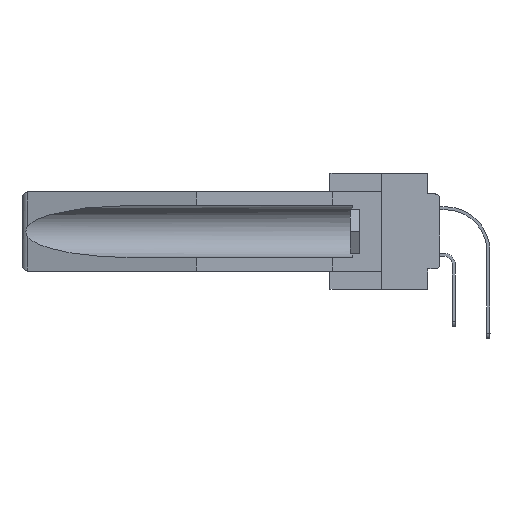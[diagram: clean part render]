
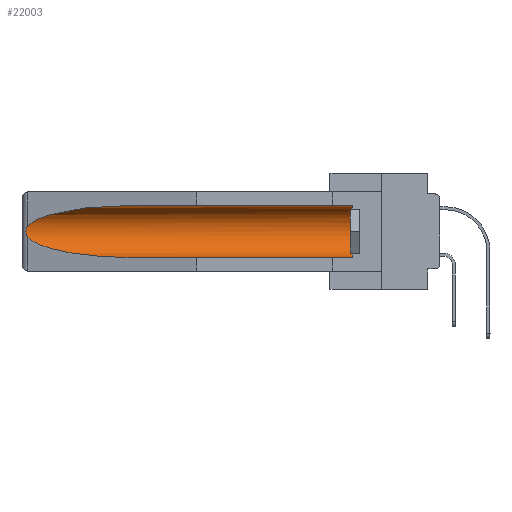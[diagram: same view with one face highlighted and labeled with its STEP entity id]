
A CAD part, left-side view. The second image highlights one B-rep face of the part: STEP entity #22003.
In plain terms, the highlighted cylindrical face has radius 2.857 mm (diameter 5.715 mm), a partial arc.
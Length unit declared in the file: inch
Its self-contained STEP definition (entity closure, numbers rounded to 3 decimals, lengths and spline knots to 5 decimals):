
#456 = AXIS2_PLACEMENT_3D ( 'NONE', #16106, #8816, #16276 ) ;
#2044 =( BOUNDED_CURVE ( )  B_SPLINE_CURVE ( 3, ( #31235, #7769, #9814, #15415 ),
 .UNSPECIFIED., .F., .T. ) 
 B_SPLINE_CURVE_WITH_KNOTS ( ( 4, 4 ),
 ( 0.1948, 1.5708 ),
 .UNSPECIFIED. ) 
 CURVE ( )  GEOMETRIC_REPRESENTATION_ITEM ( )  RATIONAL_B_SPLINE_CURVE ( ( 1., 0.848, 0.848, 1. ) ) 
 REPRESENTATION_ITEM ( '' )  );
#2384 = CARTESIAN_POINT ( 'NONE',  ( 0.26597, 1.52961, -0.15275 ) ) ;
#2824 = CARTESIAN_POINT ( 'NONE',  ( 0.155, 0.126, -0.284 ) ) ;
#3702 = EDGE_CURVE ( 'NONE', #22086, #7936, #31306, .T. ) ;
#4002 = CARTESIAN_POINT ( 'NONE',  ( 0.25451, 1.48313, -0.09465 ) ) ;
#5752 = DIRECTION ( 'NONE',  ( 0., 1., 0. ) ) ;
#6149 = ORIENTED_EDGE ( 'NONE', *, *, #23588, .T. ) ;
#6711 = ORIENTED_EDGE ( 'NONE', *, *, #3702, .F. ) ;
#6975 = CIRCLE ( 'NONE', #456, 0.1125 ) ;
#7311 = CARTESIAN_POINT ( 'NONE',  ( 0.26537, 1.52718, -0.19328 ) ) ;
#7769 = CARTESIAN_POINT ( 'NONE',  ( 0.25451, 1.48313, -0.24835 ) ) ;
#7911 =( BOUNDED_CURVE ( )  B_SPLINE_CURVE ( 3, ( #32397, #29522, #4002, #13861 ),
 .UNSPECIFIED., .F., .T. ) 
 B_SPLINE_CURVE_WITH_KNOTS ( ( 4, 4 ),
 ( 4.71239, 6.08839 ),
 .UNSPECIFIED. ) 
 CURVE ( )  GEOMETRIC_REPRESENTATION_ITEM ( )  RATIONAL_B_SPLINE_CURVE ( ( 1., 0.848, 0.848, 1. ) ) 
 REPRESENTATION_ITEM ( '' )  );
#7936 = VERTEX_POINT ( 'NONE', #20346 ) ;
#8816 = DIRECTION ( 'NONE',  ( 0., -1., 0. ) ) ;
#9614 = B_SPLINE_CURVE_WITH_KNOTS ( 'NONE', 3,
 ( #25510, #2384, #25689, #17685, #12581, #9988, #33340, #15611, #12745, #31127 ),
 .UNSPECIFIED., .F., .F.,
 ( 4, 2, 2, 2, 4 ),
 ( 0., 0.00029, 0.00058, 0.00087, 0.00117 ),
 .UNSPECIFIED. ) ;
#9814 = CARTESIAN_POINT ( 'NONE',  ( 0.21114, 1.30732, -0.284 ) ) ;
#9988 = CARTESIAN_POINT ( 'NONE',  ( 0.2675, 1.53308, -0.17534 ) ) ;
#11127 = VERTEX_POINT ( 'NONE', #25170 ) ;
#12581 = CARTESIAN_POINT ( 'NONE',  ( 0.2675, 1.53308, -0.16763 ) ) ;
#12745 = CARTESIAN_POINT ( 'NONE',  ( 0.26597, 1.5296, -0.19026 ) ) ;
#13861 = CARTESIAN_POINT ( 'NONE',  ( 0.26537, 1.52718, -0.14972 ) ) ;
#14024 = AXIS2_PLACEMENT_3D ( 'NONE', #25634, #17460, #25299 ) ;
#15058 = VECTOR ( 'NONE', #26028, 39.37008 ) ;
#15144 = EDGE_CURVE ( 'NONE', #23398, #25483, #9614, .T. ) ;
#15415 = CARTESIAN_POINT ( 'NONE',  ( 0.155, 1.07973, -0.284 ) ) ;
#15570 = CARTESIAN_POINT ( 'NONE',  ( 0.26537, 1.52718, -0.14972 ) ) ;
#15611 = CARTESIAN_POINT ( 'NONE',  ( 0.26655, 1.53094, -0.18657 ) ) ;
#15636 = CARTESIAN_POINT ( 'NONE',  ( 0.155, -0.30754, -0.284 ) ) ;
#16106 = CARTESIAN_POINT ( 'NONE',  ( 0.155, 0.126, -0.1715 ) ) ;
#16193 = VECTOR ( 'NONE', #5752, 39.37008 ) ;
#16276 = DIRECTION ( 'NONE',  ( 0., 0., 1. ) ) ;
#17460 = DIRECTION ( 'NONE',  ( 0., 1., 0. ) ) ;
#17685 = CARTESIAN_POINT ( 'NONE',  ( 0.2673, 1.5327, -0.16383 ) ) ;
#19900 = ORIENTED_EDGE ( 'NONE', *, *, #15144, .T. ) ;
#20346 = CARTESIAN_POINT ( 'NONE',  ( 0.155, 1.07973, -0.284 ) ) ;
#21026 = VERTEX_POINT ( 'NONE', #28425 ) ;
#21046 = LINE ( 'NONE', #23953, #16193 ) ;
#21612 = EDGE_CURVE ( 'NONE', #21026, #11127, #21046, .T. ) ;
#22003 = ADVANCED_FACE ( 'NONE', ( #27672 ), #24957, .F. ) ;
#22086 = VERTEX_POINT ( 'NONE', #2824 ) ;
#23398 = VERTEX_POINT ( 'NONE', #15570 ) ;
#23588 = EDGE_CURVE ( 'NONE', #11127, #23398, #7911, .T. ) ;
#23953 = CARTESIAN_POINT ( 'NONE',  ( 0.155, -0.30754, -0.059 ) ) ;
#24957 = CYLINDRICAL_SURFACE ( 'NONE', #14024, 0.1125 ) ;
#25170 = CARTESIAN_POINT ( 'NONE',  ( 0.155, 1.07973, -0.059 ) ) ;
#25299 = DIRECTION ( 'NONE',  ( 0., 0., 1. ) ) ;
#25483 = VERTEX_POINT ( 'NONE', #7311 ) ;
#25510 = CARTESIAN_POINT ( 'NONE',  ( 0.26537, 1.52718, -0.14972 ) ) ;
#25634 = CARTESIAN_POINT ( 'NONE',  ( 0.155, -0.30754, -0.1715 ) ) ;
#25689 = CARTESIAN_POINT ( 'NONE',  ( 0.26654, 1.53092, -0.15636 ) ) ;
#25864 = EDGE_CURVE ( 'NONE', #25483, #7936, #2044, .T. ) ;
#26015 = ORIENTED_EDGE ( 'NONE', *, *, #21612, .T. ) ;
#26028 = DIRECTION ( 'NONE',  ( 0., 1., 0. ) ) ;
#27672 = FACE_OUTER_BOUND ( 'NONE', #28005, .T. ) ;
#28005 = EDGE_LOOP ( 'NONE', ( #6149, #19900, #28353, #6711, #31223, #26015 ) ) ;
#28340 = EDGE_CURVE ( 'NONE', #22086, #21026, #6975, .T. ) ;
#28353 = ORIENTED_EDGE ( 'NONE', *, *, #25864, .T. ) ;
#28425 = CARTESIAN_POINT ( 'NONE',  ( 0.155, 0.126, -0.059 ) ) ;
#29522 = CARTESIAN_POINT ( 'NONE',  ( 0.21114, 1.30732, -0.059 ) ) ;
#31127 = CARTESIAN_POINT ( 'NONE',  ( 0.26537, 1.52718, -0.19328 ) ) ;
#31223 = ORIENTED_EDGE ( 'NONE', *, *, #28340, .T. ) ;
#31235 = CARTESIAN_POINT ( 'NONE',  ( 0.26537, 1.52718, -0.19328 ) ) ;
#31306 = LINE ( 'NONE', #15636, #15058 ) ;
#32397 = CARTESIAN_POINT ( 'NONE',  ( 0.155, 1.07973, -0.059 ) ) ;
#33340 = CARTESIAN_POINT ( 'NONE',  ( 0.2673, 1.53269, -0.17917 ) ) ;
